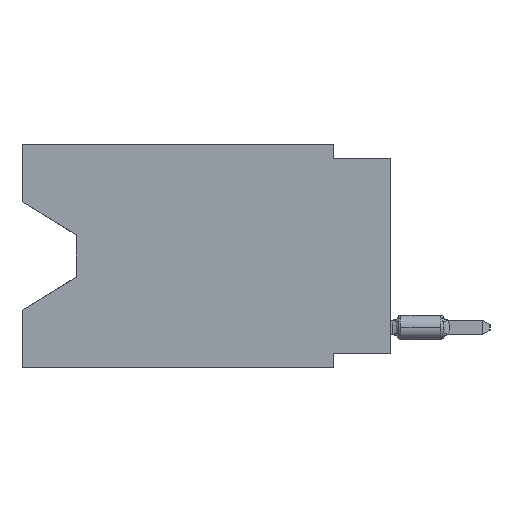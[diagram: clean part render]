
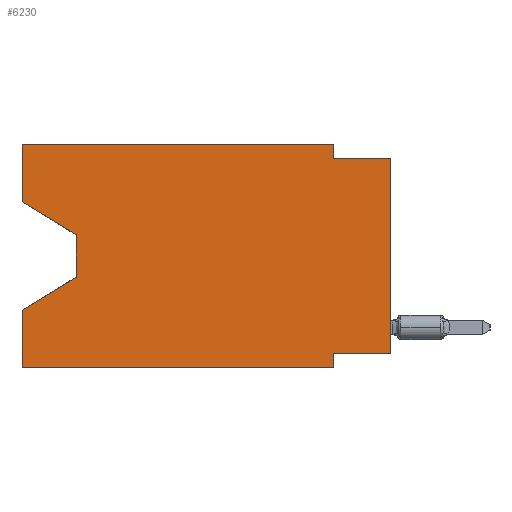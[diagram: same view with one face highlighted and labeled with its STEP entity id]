
A CAD part, left-side view. The second image highlights one B-rep face of the part: STEP entity #6230.
In plain terms, the highlighted planar face has unit normal (-1, 0, 0).
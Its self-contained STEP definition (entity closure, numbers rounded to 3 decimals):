
#155 = CARTESIAN_POINT ( 'NONE',  ( 0., 16.383, 0. ) ) ;
#425 = VERTEX_POINT ( 'NONE', #16164 ) ;
#1300 = CARTESIAN_POINT ( 'NONE',  ( 0., 16.383, 0. ) ) ;
#1664 = EDGE_CURVE ( 'NONE', #53360, #27724, #36165, .T. ) ;
#1956 = EDGE_CURVE ( 'NONE', #3253, #51543, #14744, .T. ) ;
#2872 = CARTESIAN_POINT ( 'NONE',  ( 0., 0., -0.635 ) ) ;
#3253 = VERTEX_POINT ( 'NONE', #19341 ) ;
#3707 = EDGE_CURVE ( 'NONE', #14234, #22608, #28257, .T. ) ;
#3960 = DIRECTION ( 'NONE',  ( 0., 0., -1. ) ) ;
#4303 = DIRECTION ( 'NONE',  ( 0., 0.855, -0.519 ) ) ;
#4670 = DIRECTION ( 'NONE',  ( 0., 0., 1. ) ) ;
#5116 = AXIS2_PLACEMENT_3D ( 'NONE', #155, #41594, #33446 ) ;
#5122 = VERTEX_POINT ( 'NONE', #10684 ) ;
#5557 = LINE ( 'NONE', #25774, #17518 ) ;
#5888 = DIRECTION ( 'NONE',  ( 0., 0., 1. ) ) ;
#5980 = ORIENTED_EDGE ( 'NONE', *, *, #9344, .T. ) ;
#6027 = CARTESIAN_POINT ( 'NONE',  ( 0., 13.97, -4.013 ) ) ;
#6230 = ADVANCED_FACE ( 'NONE', ( #37260 ), #53842, .F. ) ;
#6975 = EDGE_CURVE ( 'NONE', #19188, #19206, #19832, .T. ) ;
#8033 = DIRECTION ( 'NONE',  ( 0., -1., 0. ) ) ;
#8065 = DIRECTION ( 'NONE',  ( 0., 0., -1. ) ) ;
#8414 = EDGE_LOOP ( 'NONE', ( #5980, #19809, #37412, #8602, #17740, #33965, #10601, #40682, #28469, #53647, #48406, #20845 ) ) ;
#8547 = DIRECTION ( 'NONE',  ( 0., -0.855, -0.519 ) ) ;
#8602 = ORIENTED_EDGE ( 'NONE', *, *, #44759, .F. ) ;
#8818 = DIRECTION ( 'NONE',  ( 0., 0., 1. ) ) ;
#8911 = LINE ( 'NONE', #41914, #24782 ) ;
#9344 = EDGE_CURVE ( 'NONE', #53360, #19188, #33937, .T. ) ;
#9592 = CARTESIAN_POINT ( 'NONE',  ( 0., 2.54, 0. ) ) ;
#9750 = CARTESIAN_POINT ( 'NONE',  ( 0., 16.383, -2.546 ) ) ;
#10601 = ORIENTED_EDGE ( 'NONE', *, *, #1956, .F. ) ;
#10684 = CARTESIAN_POINT ( 'NONE',  ( 0., 16.383, -7.36 ) ) ;
#13455 = EDGE_CURVE ( 'NONE', #30275, #14234, #42605, .T. ) ;
#14087 = EDGE_CURVE ( 'NONE', #51543, #425, #5557, .T. ) ;
#14234 = VERTEX_POINT ( 'NONE', #14822 ) ;
#14744 = LINE ( 'NONE', #31390, #26207 ) ;
#14822 = CARTESIAN_POINT ( 'NONE',  ( 0., 2.54, -0.635 ) ) ;
#16164 = CARTESIAN_POINT ( 'NONE',  ( 0., 2.54, -9.906 ) ) ;
#17518 = VECTOR ( 'NONE', #42651, 1000. ) ;
#17740 = ORIENTED_EDGE ( 'NONE', *, *, #45220, .T. ) ;
#18465 = VECTOR ( 'NONE', #5888, 1000. ) ;
#18506 = VECTOR ( 'NONE', #8547, 1000. ) ;
#18621 = CARTESIAN_POINT ( 'NONE',  ( 0., 13.97, -5.893 ) ) ;
#19188 = VERTEX_POINT ( 'NONE', #6027 ) ;
#19206 = VERTEX_POINT ( 'NONE', #18621 ) ;
#19341 = CARTESIAN_POINT ( 'NONE',  ( 0., 0., -9.271 ) ) ;
#19809 = ORIENTED_EDGE ( 'NONE', *, *, #6975, .T. ) ;
#19832 = LINE ( 'NONE', #53577, #32124 ) ;
#20724 = CARTESIAN_POINT ( 'NONE',  ( 0., 2.54, 0. ) ) ;
#20845 = ORIENTED_EDGE ( 'NONE', *, *, #1664, .F. ) ;
#21252 = CARTESIAN_POINT ( 'NONE',  ( 0., 13.97, -5.893 ) ) ;
#22608 = VERTEX_POINT ( 'NONE', #25834 ) ;
#22945 = CARTESIAN_POINT ( 'NONE',  ( 0., 16.383, 0. ) ) ;
#23173 = VERTEX_POINT ( 'NONE', #47796 ) ;
#23814 = VECTOR ( 'NONE', #8033, 1000. ) ;
#24472 = VECTOR ( 'NONE', #4670, 1000. ) ;
#24782 = VECTOR ( 'NONE', #34291, 1000. ) ;
#25086 = LINE ( 'NONE', #21252, #40753 ) ;
#25225 = CARTESIAN_POINT ( 'NONE',  ( 0., 16.383, -2.546 ) ) ;
#25774 = CARTESIAN_POINT ( 'NONE',  ( 0., 2.54, -9.906 ) ) ;
#25834 = CARTESIAN_POINT ( 'NONE',  ( 0., 0., -0.635 ) ) ;
#26207 = VECTOR ( 'NONE', #47983, 1000. ) ;
#26875 = EDGE_CURVE ( 'NONE', #27724, #30275, #39754, .T. ) ;
#26968 = DIRECTION ( 'NONE',  ( 0., -1., 0. ) ) ;
#27604 = EDGE_CURVE ( 'NONE', #19206, #5122, #25086, .T. ) ;
#27724 = VERTEX_POINT ( 'NONE', #1300 ) ;
#28257 = LINE ( 'NONE', #2872, #23814 ) ;
#28385 = CARTESIAN_POINT ( 'NONE',  ( 0., 2.54, -9.271 ) ) ;
#28469 = ORIENTED_EDGE ( 'NONE', *, *, #3707, .F. ) ;
#30275 = VERTEX_POINT ( 'NONE', #20724 ) ;
#31278 = LINE ( 'NONE', #42995, #18465 ) ;
#31390 = CARTESIAN_POINT ( 'NONE',  ( 0., 0., -9.271 ) ) ;
#32124 = VECTOR ( 'NONE', #8065, 1000. ) ;
#33446 = DIRECTION ( 'NONE',  ( 0., 0., -1. ) ) ;
#33937 = LINE ( 'NONE', #25225, #18506 ) ;
#33965 = ORIENTED_EDGE ( 'NONE', *, *, #14087, .F. ) ;
#34291 = DIRECTION ( 'NONE',  ( 0., -1., 0. ) ) ;
#34411 = CARTESIAN_POINT ( 'NONE',  ( 0., 16.383, 0. ) ) ;
#36165 = LINE ( 'NONE', #34411, #24472 ) ;
#37260 = FACE_OUTER_BOUND ( 'NONE', #8414, .T. ) ;
#37412 = ORIENTED_EDGE ( 'NONE', *, *, #27604, .T. ) ;
#39299 = VECTOR ( 'NONE', #3960, 1000. ) ;
#39754 = LINE ( 'NONE', #47645, #51111 ) ;
#40216 = VECTOR ( 'NONE', #8818, 1000. ) ;
#40682 = ORIENTED_EDGE ( 'NONE', *, *, #40800, .T. ) ;
#40753 = VECTOR ( 'NONE', #4303, 1000. ) ;
#40800 = EDGE_CURVE ( 'NONE', #3253, #22608, #31278, .T. ) ;
#41594 = DIRECTION ( 'NONE',  ( 1., 0., 0. ) ) ;
#41914 = CARTESIAN_POINT ( 'NONE',  ( 0., 16.383, -9.906 ) ) ;
#42354 = LINE ( 'NONE', #22945, #40216 ) ;
#42605 = LINE ( 'NONE', #9592, #39299 ) ;
#42651 = DIRECTION ( 'NONE',  ( 0., 0., -1. ) ) ;
#42995 = CARTESIAN_POINT ( 'NONE',  ( 0., 0., 0. ) ) ;
#44759 = EDGE_CURVE ( 'NONE', #23173, #5122, #42354, .T. ) ;
#45220 = EDGE_CURVE ( 'NONE', #23173, #425, #8911, .T. ) ;
#47645 = CARTESIAN_POINT ( 'NONE',  ( 0., 16.383, 0. ) ) ;
#47796 = CARTESIAN_POINT ( 'NONE',  ( 0., 16.383, -9.906 ) ) ;
#47983 = DIRECTION ( 'NONE',  ( 0., 1., 0. ) ) ;
#48406 = ORIENTED_EDGE ( 'NONE', *, *, #26875, .F. ) ;
#51111 = VECTOR ( 'NONE', #26968, 1000. ) ;
#51543 = VERTEX_POINT ( 'NONE', #28385 ) ;
#53360 = VERTEX_POINT ( 'NONE', #9750 ) ;
#53577 = CARTESIAN_POINT ( 'NONE',  ( 0., 13.97, -4.013 ) ) ;
#53647 = ORIENTED_EDGE ( 'NONE', *, *, #13455, .F. ) ;
#53842 = PLANE ( 'NONE',  #5116 ) ;
